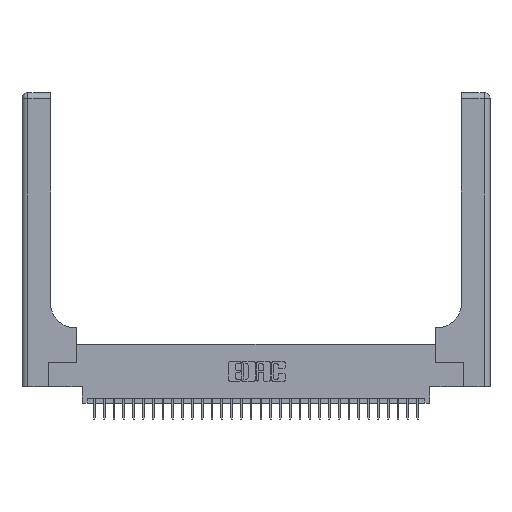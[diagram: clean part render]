
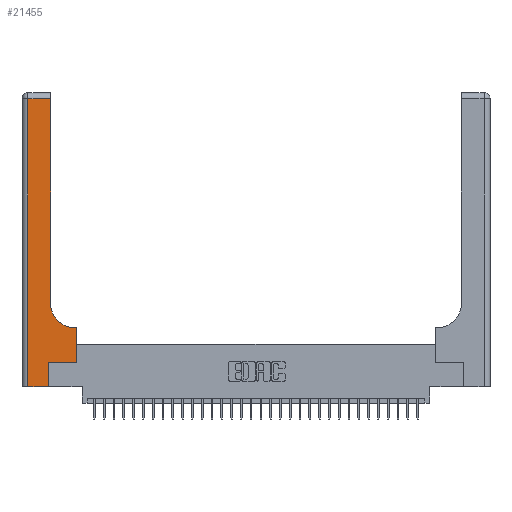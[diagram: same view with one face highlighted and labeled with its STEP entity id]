
A CAD part, top view. The second image highlights one B-rep face of the part: STEP entity #21455.
In plain terms, the highlighted planar face has unit normal (0, 0, 1).
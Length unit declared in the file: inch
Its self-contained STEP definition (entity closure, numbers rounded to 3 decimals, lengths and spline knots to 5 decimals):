
#317 = VECTOR ( 'NONE', #21598, 39.37008 ) ;
#335 = DIRECTION ( 'NONE',  ( -1., 0., 0. ) ) ;
#1444 = EDGE_LOOP ( 'NONE', ( #5287, #24345, #9777, #23910, #17797, #33103, #3222, #22016, #27924 ) ) ;
#1518 = CARTESIAN_POINT ( 'NONE',  ( 0.5585, 0.25, 0.37 ) ) ;
#2223 = AXIS2_PLACEMENT_3D ( 'NONE', #10000, #27854, #12575 ) ;
#2624 = CARTESIAN_POINT ( 'NONE',  ( 0.5585, 0.6, 0.37 ) ) ;
#3097 = LINE ( 'NONE', #25936, #9161 ) ;
#3222 = ORIENTED_EDGE ( 'NONE', *, *, #7277, .T. ) ;
#3843 = AXIS2_PLACEMENT_3D ( 'NONE', #23944, #8564, #26472 ) ;
#4053 = VECTOR ( 'NONE', #17320, 39.37008 ) ;
#4368 = CARTESIAN_POINT ( 'NONE',  ( 0.269, 0., 0.37 ) ) ;
#5026 = EDGE_CURVE ( 'NONE', #12964, #9952, #10925, .T. ) ;
#5027 = VECTOR ( 'NONE', #30579, 39.37008 ) ;
#5176 = EDGE_CURVE ( 'NONE', #9952, #31766, #25734, .T. ) ;
#5287 = ORIENTED_EDGE ( 'NONE', *, *, #10518, .T. ) ;
#6024 = VERTEX_POINT ( 'NONE', #10753 ) ;
#7277 = EDGE_CURVE ( 'NONE', #31766, #13618, #20477, .T. ) ;
#8564 = DIRECTION ( 'NONE',  ( 0., 0., -1. ) ) ;
#8859 = CARTESIAN_POINT ( 'NONE',  ( 0.269, 0., 0.37 ) ) ;
#9161 = VECTOR ( 'NONE', #335, 39.37008 ) ;
#9777 = ORIENTED_EDGE ( 'NONE', *, *, #13355, .T. ) ;
#9952 = VERTEX_POINT ( 'NONE', #27352 ) ;
#10000 = CARTESIAN_POINT ( 'NONE',  ( 0., 3., 0.37 ) ) ;
#10518 = EDGE_CURVE ( 'NONE', #20625, #11998, #20878, .T. ) ;
#10753 = CARTESIAN_POINT ( 'NONE',  ( 0.5415, 0.6, 0.37 ) ) ;
#10925 = LINE ( 'NONE', #4368, #4053 ) ;
#11998 = VERTEX_POINT ( 'NONE', #30655 ) ;
#12575 = DIRECTION ( 'NONE',  ( -1., 0., 0. ) ) ;
#12964 = VERTEX_POINT ( 'NONE', #8859 ) ;
#13080 = CARTESIAN_POINT ( 'NONE',  ( 0.06, 0., 0.37 ) ) ;
#13355 = EDGE_CURVE ( 'NONE', #30863, #16224, #32218, .T. ) ;
#13618 = VERTEX_POINT ( 'NONE', #2624 ) ;
#16224 = VERTEX_POINT ( 'NONE', #13080 ) ;
#16403 = EDGE_CURVE ( 'NONE', #6024, #20625, #31213, .T. ) ;
#16422 = CARTESIAN_POINT ( 'NONE',  ( 0.2915, 3., 0.37 ) ) ;
#16788 = CARTESIAN_POINT ( 'NONE',  ( 0.2915, 0.85, 0.37 ) ) ;
#17320 = DIRECTION ( 'NONE',  ( 0., 1., 0. ) ) ;
#17797 = ORIENTED_EDGE ( 'NONE', *, *, #5026, .T. ) ;
#17834 = EDGE_CURVE ( 'NONE', #11998, #30863, #3097, .T. ) ;
#17876 = CARTESIAN_POINT ( 'NONE',  ( 0.269, 0.25, 0.37 ) ) ;
#17946 = CARTESIAN_POINT ( 'NONE',  ( 0.06, 3., 0.37 ) ) ;
#18531 = DIRECTION ( 'NONE',  ( 1., 0., 0. ) ) ;
#18976 = VECTOR ( 'NONE', #25565, 39.37008 ) ;
#19809 = VECTOR ( 'NONE', #18531, 39.37008 ) ;
#20186 = LINE ( 'NONE', #30310, #26152 ) ;
#20477 = LINE ( 'NONE', #21357, #33152 ) ;
#20625 = VERTEX_POINT ( 'NONE', #16788 ) ;
#20878 = LINE ( 'NONE', #16422, #317 ) ;
#21357 = CARTESIAN_POINT ( 'NONE',  ( 0.5585, 0.25, 0.37 ) ) ;
#21455 = ADVANCED_FACE ( 'NONE', ( #26176 ), #22786, .F. ) ;
#21598 = DIRECTION ( 'NONE',  ( 0., 1., 0. ) ) ;
#21689 = EDGE_CURVE ( 'NONE', #16224, #12964, #28140, .T. ) ;
#22016 = ORIENTED_EDGE ( 'NONE', *, *, #31265, .T. ) ;
#22786 = PLANE ( 'NONE',  #2223 ) ;
#23910 = ORIENTED_EDGE ( 'NONE', *, *, #21689, .T. ) ;
#23944 = CARTESIAN_POINT ( 'NONE',  ( 0.5415, 0.85, 0.37 ) ) ;
#24345 = ORIENTED_EDGE ( 'NONE', *, *, #17834, .T. ) ;
#25233 = DIRECTION ( 'NONE',  ( -1., 0., 0. ) ) ;
#25565 = DIRECTION ( 'NONE',  ( 1., 0., 0. ) ) ;
#25734 = LINE ( 'NONE', #17876, #18976 ) ;
#25936 = CARTESIAN_POINT ( 'NONE',  ( 0., 2.94, 0.37 ) ) ;
#26152 = VECTOR ( 'NONE', #25233, 39.37008 ) ;
#26176 = FACE_OUTER_BOUND ( 'NONE', #1444, .T. ) ;
#26472 = DIRECTION ( 'NONE',  ( 1., 0., 0. ) ) ;
#27352 = CARTESIAN_POINT ( 'NONE',  ( 0.269, 0.25, 0.37 ) ) ;
#27854 = DIRECTION ( 'NONE',  ( 0., 0., -1. ) ) ;
#27924 = ORIENTED_EDGE ( 'NONE', *, *, #16403, .T. ) ;
#28140 = LINE ( 'NONE', #31155, #19809 ) ;
#28981 = DIRECTION ( 'NONE',  ( 0., 1., 0. ) ) ;
#30310 = CARTESIAN_POINT ( 'NONE',  ( 0.2915, 0.6, 0.37 ) ) ;
#30579 = DIRECTION ( 'NONE',  ( 0., -1., 0. ) ) ;
#30655 = CARTESIAN_POINT ( 'NONE',  ( 0.2915, 2.94, 0.37 ) ) ;
#30863 = VERTEX_POINT ( 'NONE', #32103 ) ;
#31155 = CARTESIAN_POINT ( 'NONE',  ( 0., 0., 0.37 ) ) ;
#31213 = CIRCLE ( 'NONE', #3843, 0.25 ) ;
#31265 = EDGE_CURVE ( 'NONE', #13618, #6024, #20186, .T. ) ;
#31766 = VERTEX_POINT ( 'NONE', #1518 ) ;
#32103 = CARTESIAN_POINT ( 'NONE',  ( 0.06, 2.94, 0.37 ) ) ;
#32218 = LINE ( 'NONE', #17946, #5027 ) ;
#33103 = ORIENTED_EDGE ( 'NONE', *, *, #5176, .T. ) ;
#33152 = VECTOR ( 'NONE', #28981, 39.37008 ) ;
